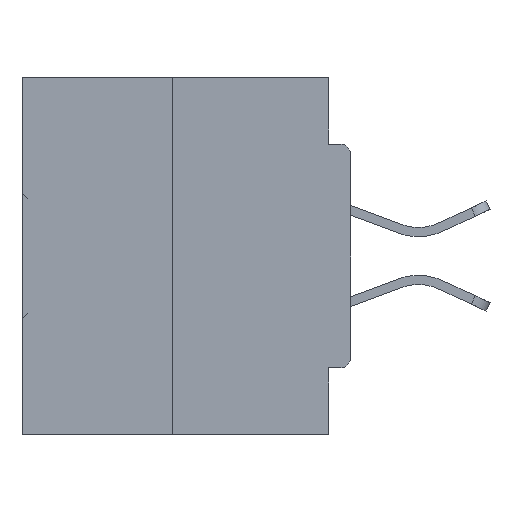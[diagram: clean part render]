
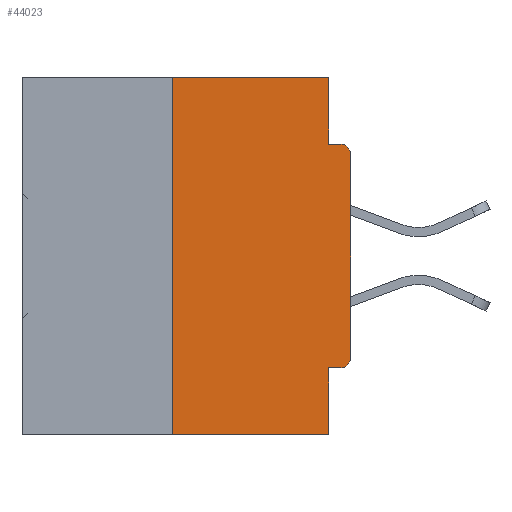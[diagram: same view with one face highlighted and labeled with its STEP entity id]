
A CAD part, left-side view. The second image highlights one B-rep face of the part: STEP entity #44023.
In plain terms, the highlighted planar face has unit normal (-1, 0, 0).
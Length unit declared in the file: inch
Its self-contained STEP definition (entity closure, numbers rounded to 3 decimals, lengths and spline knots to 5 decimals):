
#125 = ORIENTED_EDGE ( 'NONE', *, *, #1505, .F. ) ;
#478 = EDGE_CURVE ( 'NONE', #30624, #2010, #34438, .T. ) ;
#611 = EDGE_CURVE ( 'NONE', #22875, #13855, #11007, .T. ) ;
#837 = CARTESIAN_POINT ( 'NONE',  ( 0., 0.25, 0. ) ) ;
#1213 = LINE ( 'NONE', #15731, #10009 ) ;
#1505 = EDGE_CURVE ( 'NONE', #26386, #14874, #17528, .T. ) ;
#2010 = VERTEX_POINT ( 'NONE', #4965 ) ;
#3699 = DIRECTION ( 'NONE',  ( 0., -1., 0. ) ) ;
#4273 = VECTOR ( 'NONE', #17977, 39.37008 ) ;
#4965 = CARTESIAN_POINT ( 'NONE',  ( 0., 0.031, -0.5 ) ) ;
#5277 = ORIENTED_EDGE ( 'NONE', *, *, #15667, .T. ) ;
#6265 = ORIENTED_EDGE ( 'NONE', *, *, #478, .T. ) ;
#6390 = CARTESIAN_POINT ( 'NONE',  ( 0., 0., 0. ) ) ;
#8819 = FACE_OUTER_BOUND ( 'NONE', #23947, .T. ) ;
#9293 = EDGE_CURVE ( 'NONE', #17119, #29443, #43752, .T. ) ;
#10009 = VECTOR ( 'NONE', #30297, 39.37008 ) ;
#11007 = LINE ( 'NONE', #32264, #13152 ) ;
#11825 = CARTESIAN_POINT ( 'NONE',  ( 0., 0.031, -0.5 ) ) ;
#12059 = DIRECTION ( 'NONE',  ( 0., 0., -1. ) ) ;
#12157 = PLANE ( 'NONE',  #24079 ) ;
#12389 = VECTOR ( 'NONE', #16766, 39.37008 ) ;
#12479 = LINE ( 'NONE', #837, #16609 ) ;
#12691 = CIRCLE ( 'NONE', #36288, 0.015 ) ;
#13026 = VERTEX_POINT ( 'NONE', #16622 ) ;
#13152 = VECTOR ( 'NONE', #28458, 39.37008 ) ;
#13766 = DIRECTION ( 'NONE',  ( 0., 0., 1. ) ) ;
#13855 = VERTEX_POINT ( 'NONE', #23872 ) ;
#14721 = ORIENTED_EDGE ( 'NONE', *, *, #37172, .F. ) ;
#14874 = VERTEX_POINT ( 'NONE', #38698 ) ;
#15667 = EDGE_CURVE ( 'NONE', #17119, #13026, #12691, .T. ) ;
#15731 = CARTESIAN_POINT ( 'NONE',  ( 0., 0.031, 0. ) ) ;
#16609 = VECTOR ( 'NONE', #26818, 39.37008 ) ;
#16622 = CARTESIAN_POINT ( 'NONE',  ( 0., 0., -0.3915 ) ) ;
#16766 = DIRECTION ( 'NONE',  ( 0., -1., 0. ) ) ;
#17005 = CARTESIAN_POINT ( 'NONE',  ( 0., 0.46, -0.5 ) ) ;
#17119 = VERTEX_POINT ( 'NONE', #26137 ) ;
#17528 = LINE ( 'NONE', #36364, #33787 ) ;
#17562 = CARTESIAN_POINT ( 'NONE',  ( 0., 0.031, -0.4065 ) ) ;
#17692 = ORIENTED_EDGE ( 'NONE', *, *, #44739, .F. ) ;
#17732 = CARTESIAN_POINT ( 'NONE',  ( 0., 0.031, -0.0935 ) ) ;
#17977 = DIRECTION ( 'NONE',  ( 0., 1., 0. ) ) ;
#18834 = CARTESIAN_POINT ( 'NONE',  ( 0., 0.46, 0. ) ) ;
#18978 = DIRECTION ( 'NONE',  ( 0., 0., -1. ) ) ;
#19684 = DIRECTION ( 'NONE',  ( -1., 0., 0. ) ) ;
#21517 = VERTEX_POINT ( 'NONE', #25661 ) ;
#21940 = CIRCLE ( 'NONE', #32613, 0.015 ) ;
#22605 = CARTESIAN_POINT ( 'NONE',  ( 0., 0.015, -0.3915 ) ) ;
#22875 = VERTEX_POINT ( 'NONE', #23239 ) ;
#23174 = VECTOR ( 'NONE', #13766, 39.37008 ) ;
#23239 = CARTESIAN_POINT ( 'NONE',  ( 0., 0.25, 0. ) ) ;
#23872 = CARTESIAN_POINT ( 'NONE',  ( 0., 0.031, 0. ) ) ;
#23947 = EDGE_LOOP ( 'NONE', ( #33644, #17692, #6265, #39943, #24821, #5277, #38901, #25743, #125, #14721 ) ) ;
#24079 = AXIS2_PLACEMENT_3D ( 'NONE', #18834, #33398, #26723 ) ;
#24821 = ORIENTED_EDGE ( 'NONE', *, *, #9293, .F. ) ;
#25661 = CARTESIAN_POINT ( 'NONE',  ( 0., 0., -0.1085 ) ) ;
#25743 = ORIENTED_EDGE ( 'NONE', *, *, #27338, .T. ) ;
#26137 = CARTESIAN_POINT ( 'NONE',  ( 0., 0.015, -0.4065 ) ) ;
#26386 = VERTEX_POINT ( 'NONE', #17732 ) ;
#26723 = DIRECTION ( 'NONE',  ( 0., 0., -1. ) ) ;
#26749 = CARTESIAN_POINT ( 'NONE',  ( 0., 0.25, -0.5 ) ) ;
#26818 = DIRECTION ( 'NONE',  ( 0., 0., 1. ) ) ;
#27338 = EDGE_CURVE ( 'NONE', #21517, #14874, #21940, .T. ) ;
#27348 = VECTOR ( 'NONE', #18978, 39.37008 ) ;
#27437 = EDGE_CURVE ( 'NONE', #29443, #2010, #37105, .T. ) ;
#28458 = DIRECTION ( 'NONE',  ( 0., -1., 0. ) ) ;
#29443 = VERTEX_POINT ( 'NONE', #17562 ) ;
#30297 = DIRECTION ( 'NONE',  ( 0., 0., -1. ) ) ;
#30624 = VERTEX_POINT ( 'NONE', #26749 ) ;
#30665 = CARTESIAN_POINT ( 'NONE',  ( 0., 0.015, -0.1085 ) ) ;
#32264 = CARTESIAN_POINT ( 'NONE',  ( 0., 0.46, 0. ) ) ;
#32613 = AXIS2_PLACEMENT_3D ( 'NONE', #30665, #19684, #12059 ) ;
#33398 = DIRECTION ( 'NONE',  ( 1., 0., 0. ) ) ;
#33644 = ORIENTED_EDGE ( 'NONE', *, *, #611, .F. ) ;
#33787 = VECTOR ( 'NONE', #3699, 39.37008 ) ;
#34438 = LINE ( 'NONE', #17005, #12389 ) ;
#36288 = AXIS2_PLACEMENT_3D ( 'NONE', #22605, #44559, #37156 ) ;
#36364 = CARTESIAN_POINT ( 'NONE',  ( 0., 0., -0.0935 ) ) ;
#37057 = CARTESIAN_POINT ( 'NONE',  ( 0., 0., -0.4065 ) ) ;
#37105 = LINE ( 'NONE', #11825, #27348 ) ;
#37156 = DIRECTION ( 'NONE',  ( 0., 0., -1. ) ) ;
#37172 = EDGE_CURVE ( 'NONE', #13855, #26386, #1213, .T. ) ;
#38698 = CARTESIAN_POINT ( 'NONE',  ( 0., 0.015, -0.0935 ) ) ;
#38901 = ORIENTED_EDGE ( 'NONE', *, *, #40590, .T. ) ;
#39062 = LINE ( 'NONE', #6390, #23174 ) ;
#39943 = ORIENTED_EDGE ( 'NONE', *, *, #27437, .F. ) ;
#40590 = EDGE_CURVE ( 'NONE', #13026, #21517, #39062, .T. ) ;
#43752 = LINE ( 'NONE', #37057, #4273 ) ;
#44023 = ADVANCED_FACE ( 'NONE', ( #8819 ), #12157, .F. ) ;
#44559 = DIRECTION ( 'NONE',  ( -1., 0., 0. ) ) ;
#44739 = EDGE_CURVE ( 'NONE', #30624, #22875, #12479, .T. ) ;
